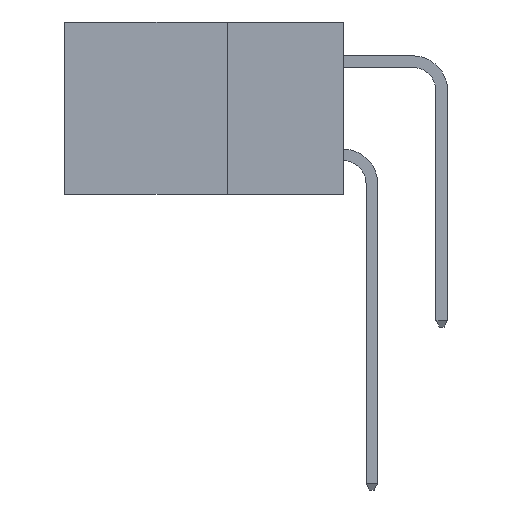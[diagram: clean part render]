
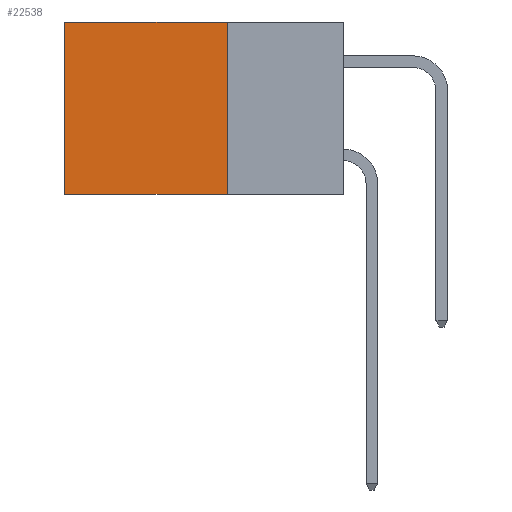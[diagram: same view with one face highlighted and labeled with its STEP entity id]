
A CAD part, left-side view. The second image highlights one B-rep face of the part: STEP entity #22538.
In plain terms, the highlighted planar face has unit normal (-1, 0, 0).
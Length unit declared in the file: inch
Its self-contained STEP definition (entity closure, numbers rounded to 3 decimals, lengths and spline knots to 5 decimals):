
#557 = EDGE_CURVE ( 'NONE', #2525, #25364, #11723, .T. ) ;
#1364 = CARTESIAN_POINT ( 'NONE',  ( 0.2615, 0.6, 0. ) ) ;
#1478 = ORIENTED_EDGE ( 'NONE', *, *, #23155, .T. ) ;
#2525 = VERTEX_POINT ( 'NONE', #21560 ) ;
#3873 = EDGE_CURVE ( 'NONE', #25126, #24244, #20120, .T. ) ;
#4001 = DIRECTION ( 'NONE',  ( 0., 0., -1. ) ) ;
#4933 = CARTESIAN_POINT ( 'NONE',  ( 0.2615, 0.25, -0.37 ) ) ;
#6729 = ORIENTED_EDGE ( 'NONE', *, *, #3873, .F. ) ;
#6854 = CARTESIAN_POINT ( 'NONE',  ( 0.2615, 0.6, -0.37 ) ) ;
#7081 = PLANE ( 'NONE',  #18630 ) ;
#8223 = VECTOR ( 'NONE', #20241, 39.37008 ) ;
#9232 = DIRECTION ( 'NONE',  ( 1., 0., 0. ) ) ;
#10159 = CARTESIAN_POINT ( 'NONE',  ( 0.2615, 0.6, -0.37 ) ) ;
#11723 = LINE ( 'NONE', #14061, #22263 ) ;
#12495 = CARTESIAN_POINT ( 'NONE',  ( 0.2615, 0.25, -0.37 ) ) ;
#12576 = DIRECTION ( 'NONE',  ( 0., 1., 0. ) ) ;
#13004 = EDGE_CURVE ( 'NONE', #2525, #25126, #26294, .T. ) ;
#13148 = EDGE_LOOP ( 'NONE', ( #1478, #6729, #14554, #26274 ) ) ;
#13302 = CARTESIAN_POINT ( 'NONE',  ( 0.2615, 0.25, -0.37 ) ) ;
#14061 = CARTESIAN_POINT ( 'NONE',  ( 0.2615, 0.25, 0. ) ) ;
#14554 = ORIENTED_EDGE ( 'NONE', *, *, #13004, .F. ) ;
#15302 = FACE_OUTER_BOUND ( 'NONE', #13148, .T. ) ;
#17572 = VECTOR ( 'NONE', #21651, 39.37008 ) ;
#18630 = AXIS2_PLACEMENT_3D ( 'NONE', #4933, #9232, #23996 ) ;
#20120 = LINE ( 'NONE', #20488, #8223 ) ;
#20241 = DIRECTION ( 'NONE',  ( 0., 1., 0. ) ) ;
#20488 = CARTESIAN_POINT ( 'NONE',  ( 0.2615, 0.25, -0.37 ) ) ;
#20671 = VECTOR ( 'NONE', #4001, 39.37008 ) ;
#21560 = CARTESIAN_POINT ( 'NONE',  ( 0.2615, 0.25, 0. ) ) ;
#21651 = DIRECTION ( 'NONE',  ( 0., 0., -1. ) ) ;
#22263 = VECTOR ( 'NONE', #12576, 39.37008 ) ;
#22489 = LINE ( 'NONE', #6854, #17572 ) ;
#22538 = ADVANCED_FACE ( 'NONE', ( #15302 ), #7081, .F. ) ;
#23155 = EDGE_CURVE ( 'NONE', #25364, #24244, #22489, .T. ) ;
#23996 = DIRECTION ( 'NONE',  ( 0., 0., -1. ) ) ;
#24244 = VERTEX_POINT ( 'NONE', #10159 ) ;
#25126 = VERTEX_POINT ( 'NONE', #13302 ) ;
#25364 = VERTEX_POINT ( 'NONE', #1364 ) ;
#26274 = ORIENTED_EDGE ( 'NONE', *, *, #557, .T. ) ;
#26294 = LINE ( 'NONE', #12495, #20671 ) ;
